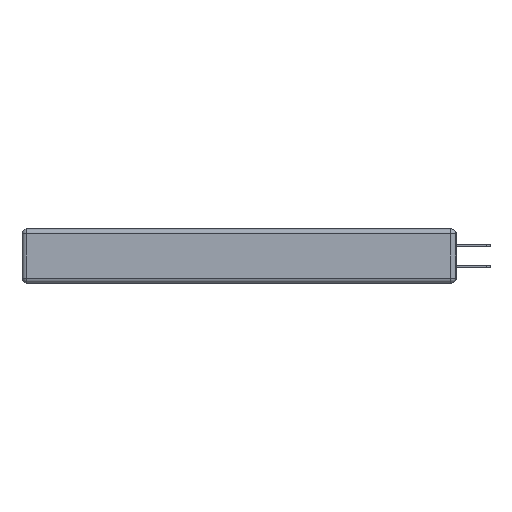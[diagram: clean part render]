
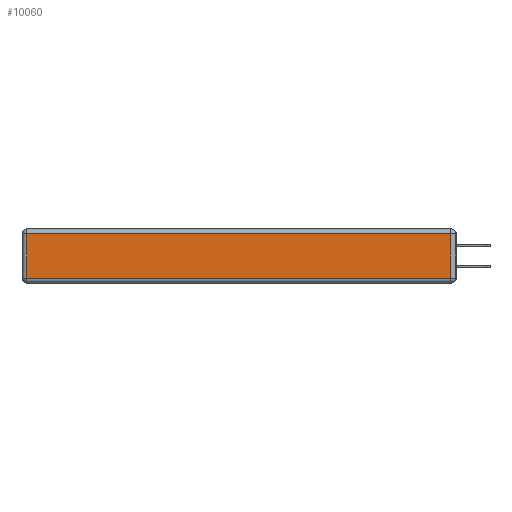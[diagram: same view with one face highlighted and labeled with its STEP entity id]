
A CAD part, left-side view. The second image highlights one B-rep face of the part: STEP entity #10060.
In plain terms, the highlighted planar face has unit normal (-1, 0, 0).
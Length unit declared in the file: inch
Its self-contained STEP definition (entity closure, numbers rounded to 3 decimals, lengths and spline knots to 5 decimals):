
#797 = LINE ( 'NONE', #14463, #17369 ) ;
#1096 = ORIENTED_EDGE ( 'NONE', *, *, #2336, .T. ) ;
#1175 = VECTOR ( 'NONE', #7299, 39.37008 ) ;
#1610 = DIRECTION ( 'NONE',  ( 0., 1., 0. ) ) ;
#2336 = EDGE_CURVE ( 'NONE', #8428, #6149, #12708, .T. ) ;
#3261 = VECTOR ( 'NONE', #3717, 39.37008 ) ;
#3717 = DIRECTION ( 'NONE',  ( 0., 0., -1. ) ) ;
#4317 = PLANE ( 'NONE',  #6171 ) ;
#4452 = EDGE_CURVE ( 'NONE', #10583, #8428, #12438, .T. ) ;
#5595 = CARTESIAN_POINT ( 'NONE',  ( 0., 2.72, -0.03 ) ) ;
#6149 = VERTEX_POINT ( 'NONE', #10410 ) ;
#6171 = AXIS2_PLACEMENT_3D ( 'NONE', #6992, #13659, #15146 ) ;
#6172 = ORIENTED_EDGE ( 'NONE', *, *, #4452, .T. ) ;
#6499 = VECTOR ( 'NONE', #1610, 39.37008 ) ;
#6717 = EDGE_LOOP ( 'NONE', ( #1096, #13695, #13709, #6172 ) ) ;
#6904 = CARTESIAN_POINT ( 'NONE',  ( 0., 0.03, -0.03 ) ) ;
#6992 = CARTESIAN_POINT ( 'NONE',  ( 0., 0., -0.343 ) ) ;
#7299 = DIRECTION ( 'NONE',  ( 0., -1., 0. ) ) ;
#8170 = LINE ( 'NONE', #9671, #6499 ) ;
#8224 = EDGE_CURVE ( 'NONE', #6149, #14612, #797, .T. ) ;
#8428 = VERTEX_POINT ( 'NONE', #16908 ) ;
#9671 = CARTESIAN_POINT ( 'NONE',  ( 0., 2.75, -0.03 ) ) ;
#10060 = ADVANCED_FACE ( 'NONE', ( #11834 ), #4317, .T. ) ;
#10385 = CARTESIAN_POINT ( 'NONE',  ( 0., 2.72, -0.343 ) ) ;
#10410 = CARTESIAN_POINT ( 'NONE',  ( 0., 0.03, -0.313 ) ) ;
#10583 = VERTEX_POINT ( 'NONE', #5595 ) ;
#11834 = FACE_OUTER_BOUND ( 'NONE', #6717, .T. ) ;
#12438 = LINE ( 'NONE', #10385, #3261 ) ;
#12708 = LINE ( 'NONE', #15465, #1175 ) ;
#13659 = DIRECTION ( 'NONE',  ( -1., 0., 0. ) ) ;
#13695 = ORIENTED_EDGE ( 'NONE', *, *, #8224, .T. ) ;
#13709 = ORIENTED_EDGE ( 'NONE', *, *, #16183, .T. ) ;
#14463 = CARTESIAN_POINT ( 'NONE',  ( 0., 0.03, -0.343 ) ) ;
#14612 = VERTEX_POINT ( 'NONE', #6904 ) ;
#15146 = DIRECTION ( 'NONE',  ( 0., 0., 1. ) ) ;
#15465 = CARTESIAN_POINT ( 'NONE',  ( 0., 0., -0.313 ) ) ;
#15874 = DIRECTION ( 'NONE',  ( 0., 0., 1. ) ) ;
#16183 = EDGE_CURVE ( 'NONE', #14612, #10583, #8170, .T. ) ;
#16908 = CARTESIAN_POINT ( 'NONE',  ( 0., 2.72, -0.313 ) ) ;
#17369 = VECTOR ( 'NONE', #15874, 39.37008 ) ;
